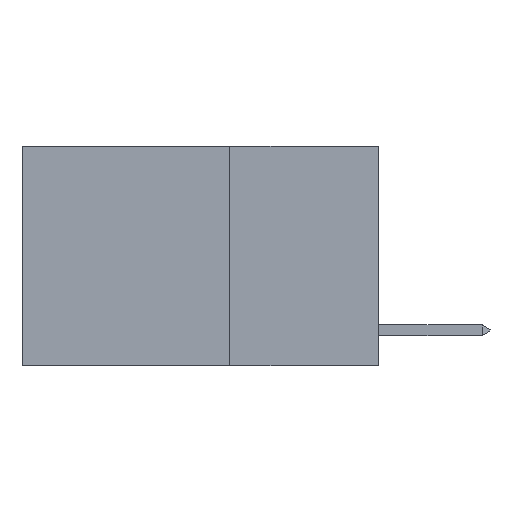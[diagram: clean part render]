
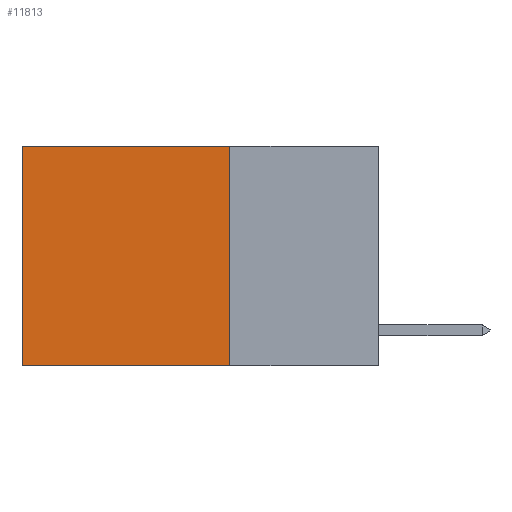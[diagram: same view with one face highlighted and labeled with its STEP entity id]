
A CAD part, left-side view. The second image highlights one B-rep face of the part: STEP entity #11813.
In plain terms, the highlighted planar face has unit normal (-1, 0, 0).
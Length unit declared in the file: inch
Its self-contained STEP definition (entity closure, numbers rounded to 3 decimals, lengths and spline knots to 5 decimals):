
#290 = DIRECTION ( 'NONE',  ( 0., 0., -1. ) ) ;
#621 = CARTESIAN_POINT ( 'NONE',  ( 0.2625, 0.25, 0. ) ) ;
#903 = DIRECTION ( 'NONE',  ( 1., 0., 0. ) ) ;
#1119 = VECTOR ( 'NONE', #11608, 39.37008 ) ;
#1617 = CARTESIAN_POINT ( 'NONE',  ( 0.2625, 0.25, 0. ) ) ;
#1754 = VECTOR ( 'NONE', #290, 39.37008 ) ;
#1785 = CARTESIAN_POINT ( 'NONE',  ( 0.2625, 0.25, -0.37 ) ) ;
#1886 = EDGE_CURVE ( 'NONE', #15551, #8663, #7396, .T. ) ;
#2141 = CARTESIAN_POINT ( 'NONE',  ( 0.2625, 0.25, 0. ) ) ;
#3719 = ORIENTED_EDGE ( 'NONE', *, *, #5507, .T. ) ;
#3770 = LINE ( 'NONE', #2141, #9895 ) ;
#4068 = EDGE_CURVE ( 'NONE', #4583, #15551, #10880, .T. ) ;
#4583 = VERTEX_POINT ( 'NONE', #1617 ) ;
#4613 = EDGE_LOOP ( 'NONE', ( #6953, #9373, #5407, #3719 ) ) ;
#4743 = LINE ( 'NONE', #10295, #1754 ) ;
#4818 = VECTOR ( 'NONE', #8141, 39.37008 ) ;
#5233 = EDGE_CURVE ( 'NONE', #15285, #8663, #4743, .T. ) ;
#5407 = ORIENTED_EDGE ( 'NONE', *, *, #4068, .F. ) ;
#5490 = CARTESIAN_POINT ( 'NONE',  ( 0.2625, 0.6, -0.37 ) ) ;
#5507 = EDGE_CURVE ( 'NONE', #4583, #15285, #3770, .T. ) ;
#5812 = CARTESIAN_POINT ( 'NONE',  ( 0.2625, 0.25, -0.37 ) ) ;
#5936 = DIRECTION ( 'NONE',  ( 0., 1., 0. ) ) ;
#6953 = ORIENTED_EDGE ( 'NONE', *, *, #5233, .T. ) ;
#7159 = PLANE ( 'NONE',  #12017 ) ;
#7396 = LINE ( 'NONE', #1785, #1119 ) ;
#8141 = DIRECTION ( 'NONE',  ( 0., 0., -1. ) ) ;
#8477 = CARTESIAN_POINT ( 'NONE',  ( 0.2625, 0.6, 0. ) ) ;
#8663 = VERTEX_POINT ( 'NONE', #5490 ) ;
#9373 = ORIENTED_EDGE ( 'NONE', *, *, #1886, .F. ) ;
#9605 = DIRECTION ( 'NONE',  ( 0., 0., -1. ) ) ;
#9895 = VECTOR ( 'NONE', #5936, 39.37008 ) ;
#10295 = CARTESIAN_POINT ( 'NONE',  ( 0.2625, 0.6, 0. ) ) ;
#10880 = LINE ( 'NONE', #621, #4818 ) ;
#11608 = DIRECTION ( 'NONE',  ( 0., 1., 0. ) ) ;
#11813 = ADVANCED_FACE ( 'NONE', ( #12494 ), #7159, .F. ) ;
#12017 = AXIS2_PLACEMENT_3D ( 'NONE', #15636, #903, #9605 ) ;
#12494 = FACE_OUTER_BOUND ( 'NONE', #4613, .T. ) ;
#15285 = VERTEX_POINT ( 'NONE', #8477 ) ;
#15551 = VERTEX_POINT ( 'NONE', #5812 ) ;
#15636 = CARTESIAN_POINT ( 'NONE',  ( 0.2625, 0.25, 0. ) ) ;
